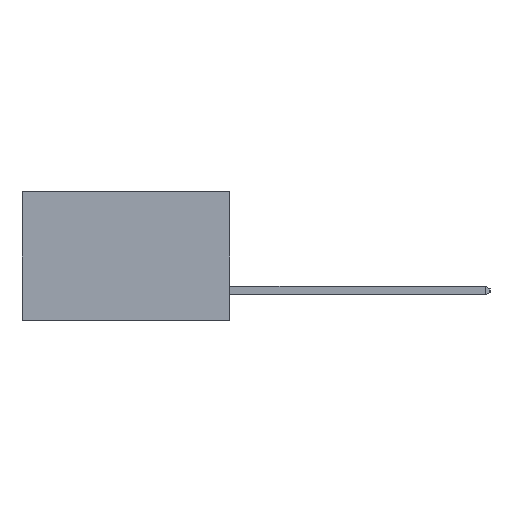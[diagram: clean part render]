
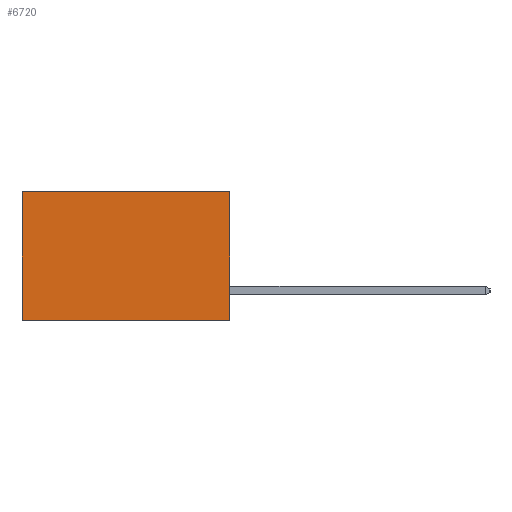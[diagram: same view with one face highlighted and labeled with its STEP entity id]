
A CAD part, left-side view. The second image highlights one B-rep face of the part: STEP entity #6720.
In plain terms, the highlighted planar face has unit normal (-1, 0, 0).
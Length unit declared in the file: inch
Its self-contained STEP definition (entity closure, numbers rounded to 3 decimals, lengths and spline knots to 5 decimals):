
#601 = VECTOR ( 'NONE', #11684, 39.37008 ) ;
#1552 = EDGE_CURVE ( 'NONE', #10967, #18458, #17207, .T. ) ;
#1938 = ORIENTED_EDGE ( 'NONE', *, *, #1552, .T. ) ;
#2113 = ORIENTED_EDGE ( 'NONE', *, *, #4250, .F. ) ;
#2484 = VECTOR ( 'NONE', #7187, 39.37008 ) ;
#2570 = EDGE_CURVE ( 'NONE', #3801, #22580, #14737, .T. ) ;
#3564 = VECTOR ( 'NONE', #18471, 39.37008 ) ;
#3726 = DIRECTION ( 'NONE',  ( 0., 0., -1. ) ) ;
#3795 = DIRECTION ( 'NONE',  ( 1., 0., 0. ) ) ;
#3801 = VERTEX_POINT ( 'NONE', #10997 ) ;
#3908 = PLANE ( 'NONE',  #16428 ) ;
#4250 = EDGE_CURVE ( 'NONE', #10967, #3801, #16491, .T. ) ;
#4625 = EDGE_LOOP ( 'NONE', ( #11428, #6448, #2113, #1938 ) ) ;
#4753 = CARTESIAN_POINT ( 'NONE',  ( 0.2615, 0., -0.37 ) ) ;
#6202 = CARTESIAN_POINT ( 'NONE',  ( 0.2615, 0., 0. ) ) ;
#6448 = ORIENTED_EDGE ( 'NONE', *, *, #2570, .F. ) ;
#6571 = FACE_OUTER_BOUND ( 'NONE', #4625, .T. ) ;
#6720 = ADVANCED_FACE ( 'NONE', ( #6571 ), #3908, .F. ) ;
#6832 = EDGE_CURVE ( 'NONE', #18458, #22580, #23431, .T. ) ;
#7187 = DIRECTION ( 'NONE',  ( 0., 1., 0. ) ) ;
#7821 = CARTESIAN_POINT ( 'NONE',  ( 0.2615, 0.6, 0. ) ) ;
#8497 = DIRECTION ( 'NONE',  ( 0., 0., -1. ) ) ;
#9689 = CARTESIAN_POINT ( 'NONE',  ( 0.2615, 0., -0.37 ) ) ;
#10967 = VERTEX_POINT ( 'NONE', #22850 ) ;
#10997 = CARTESIAN_POINT ( 'NONE',  ( 0.2615, 0., -0.37 ) ) ;
#11294 = VECTOR ( 'NONE', #8497, 39.37008 ) ;
#11428 = ORIENTED_EDGE ( 'NONE', *, *, #6832, .T. ) ;
#11663 = CARTESIAN_POINT ( 'NONE',  ( 0.2615, 0., -0.37 ) ) ;
#11684 = DIRECTION ( 'NONE',  ( 0., 1., 0. ) ) ;
#14737 = LINE ( 'NONE', #11663, #601 ) ;
#16428 = AXIS2_PLACEMENT_3D ( 'NONE', #4753, #3795, #3726 ) ;
#16491 = LINE ( 'NONE', #9689, #11294 ) ;
#17207 = LINE ( 'NONE', #6202, #2484 ) ;
#18458 = VERTEX_POINT ( 'NONE', #7821 ) ;
#18471 = DIRECTION ( 'NONE',  ( 0., 0., -1. ) ) ;
#19343 = CARTESIAN_POINT ( 'NONE',  ( 0.2615, 0.6, -0.37 ) ) ;
#20515 = CARTESIAN_POINT ( 'NONE',  ( 0.2615, 0.6, -0.37 ) ) ;
#22580 = VERTEX_POINT ( 'NONE', #20515 ) ;
#22850 = CARTESIAN_POINT ( 'NONE',  ( 0.2615, 0., 0. ) ) ;
#23431 = LINE ( 'NONE', #19343, #3564 ) ;
